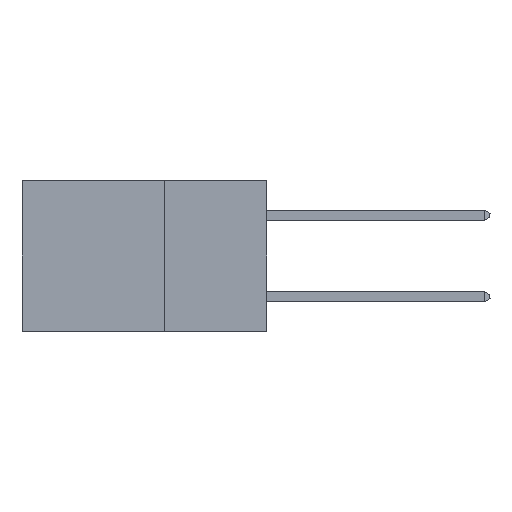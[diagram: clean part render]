
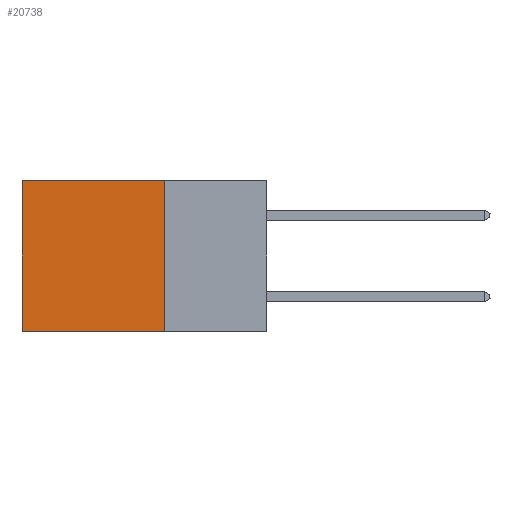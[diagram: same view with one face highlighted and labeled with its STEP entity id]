
A CAD part, left-side view. The second image highlights one B-rep face of the part: STEP entity #20738.
In plain terms, the highlighted planar face has unit normal (-1, 0, 0).
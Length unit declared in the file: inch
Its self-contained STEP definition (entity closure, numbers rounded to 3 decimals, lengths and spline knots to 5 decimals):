
#39 = CARTESIAN_POINT ( 'NONE',  ( 0.2875, 0.25, 0. ) ) ;
#152 = DIRECTION ( 'NONE',  ( 0., 0., -1. ) ) ;
#245 = EDGE_CURVE ( 'NONE', #19656, #16483, #5565, .T. ) ;
#1281 = CARTESIAN_POINT ( 'NONE',  ( 0.2875, 0.25, -0.37 ) ) ;
#1651 = CARTESIAN_POINT ( 'NONE',  ( 0.2875, 0.25, 0. ) ) ;
#1876 = EDGE_CURVE ( 'NONE', #12619, #19656, #21315, .T. ) ;
#1898 = DIRECTION ( 'NONE',  ( 0., 0., -1. ) ) ;
#2582 = AXIS2_PLACEMENT_3D ( 'NONE', #39, #12504, #1898 ) ;
#2966 = DIRECTION ( 'NONE',  ( 0., 1., 0. ) ) ;
#3459 = VECTOR ( 'NONE', #152, 39.37008 ) ;
#3480 = VECTOR ( 'NONE', #2966, 39.37008 ) ;
#4293 = CARTESIAN_POINT ( 'NONE',  ( 0.2875, 0.6, -0.37 ) ) ;
#5565 = LINE ( 'NONE', #12285, #14290 ) ;
#5860 = ORIENTED_EDGE ( 'NONE', *, *, #245, .T. ) ;
#6027 = EDGE_CURVE ( 'NONE', #15022, #16483, #21384, .T. ) ;
#7794 = VECTOR ( 'NONE', #12184, 39.37008 ) ;
#8471 = ORIENTED_EDGE ( 'NONE', *, *, #6027, .F. ) ;
#9331 = CARTESIAN_POINT ( 'NONE',  ( 0.2875, 0.6, 0. ) ) ;
#9736 = FACE_OUTER_BOUND ( 'NONE', #21998, .T. ) ;
#9943 = ORIENTED_EDGE ( 'NONE', *, *, #16969, .F. ) ;
#10797 = PLANE ( 'NONE',  #2582 ) ;
#12184 = DIRECTION ( 'NONE',  ( 0., 1., 0. ) ) ;
#12285 = CARTESIAN_POINT ( 'NONE',  ( 0.2875, 0.6, 0. ) ) ;
#12356 = DIRECTION ( 'NONE',  ( 0., 0., -1. ) ) ;
#12504 = DIRECTION ( 'NONE',  ( 1., 0., 0. ) ) ;
#12619 = VERTEX_POINT ( 'NONE', #1651 ) ;
#14290 = VECTOR ( 'NONE', #12356, 39.37008 ) ;
#14333 = CARTESIAN_POINT ( 'NONE',  ( 0.2875, 0.25, 0. ) ) ;
#15022 = VERTEX_POINT ( 'NONE', #1281 ) ;
#15277 = CARTESIAN_POINT ( 'NONE',  ( 0.2875, 0.25, 0. ) ) ;
#16483 = VERTEX_POINT ( 'NONE', #4293 ) ;
#16969 = EDGE_CURVE ( 'NONE', #12619, #15022, #21299, .T. ) ;
#18906 = CARTESIAN_POINT ( 'NONE',  ( 0.2875, 0.25, -0.37 ) ) ;
#19656 = VERTEX_POINT ( 'NONE', #9331 ) ;
#20738 = ADVANCED_FACE ( 'NONE', ( #9736 ), #10797, .F. ) ;
#21299 = LINE ( 'NONE', #14333, #3459 ) ;
#21315 = LINE ( 'NONE', #15277, #3480 ) ;
#21384 = LINE ( 'NONE', #18906, #7794 ) ;
#21998 = EDGE_LOOP ( 'NONE', ( #5860, #8471, #9943, #22227 ) ) ;
#22227 = ORIENTED_EDGE ( 'NONE', *, *, #1876, .T. ) ;
